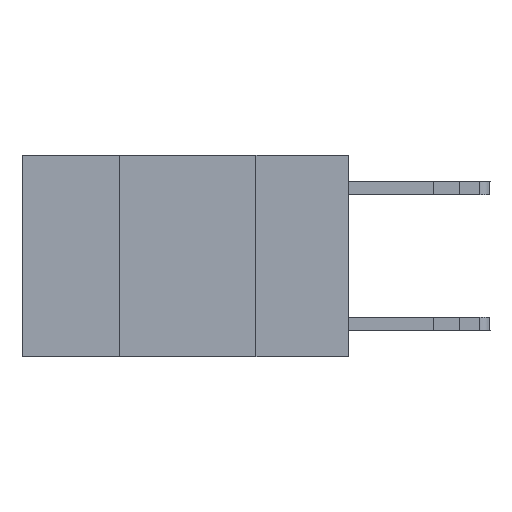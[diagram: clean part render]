
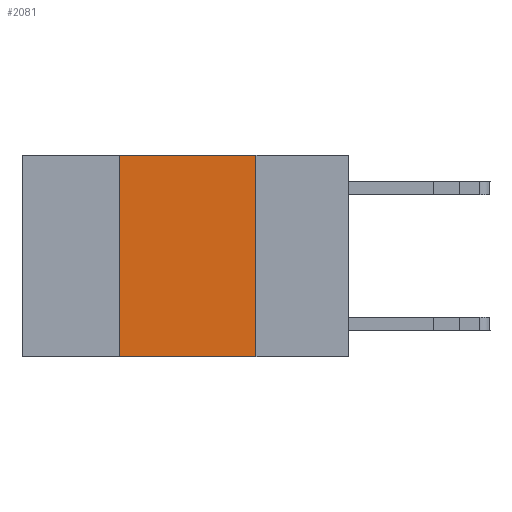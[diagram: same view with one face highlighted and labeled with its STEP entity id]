
A CAD part, left-side view. The second image highlights one B-rep face of the part: STEP entity #2081.
In plain terms, the highlighted planar face has unit normal (-1, 0, 0).
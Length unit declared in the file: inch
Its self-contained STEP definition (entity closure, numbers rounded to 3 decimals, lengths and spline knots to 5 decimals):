
#40 = LINE ( 'NONE', #5530, #3057 ) ;
#93 = CARTESIAN_POINT ( 'NONE',  ( 0., 0.17, -0.37 ) ) ;
#154 = VECTOR ( 'NONE', #2727, 39.37008 ) ;
#348 = EDGE_LOOP ( 'NONE', ( #658, #7552, #931, #5049 ) ) ;
#658 = ORIENTED_EDGE ( 'NONE', *, *, #816, .F. ) ;
#706 = VECTOR ( 'NONE', #5770, 39.37008 ) ;
#811 = DIRECTION ( 'NONE',  ( 1., 0., 0. ) ) ;
#816 = EDGE_CURVE ( 'NONE', #6976, #3836, #6432, .T. ) ;
#931 = ORIENTED_EDGE ( 'NONE', *, *, #13270, .F. ) ;
#2059 = DIRECTION ( 'NONE',  ( 0., 0., -1. ) ) ;
#2081 = ADVANCED_FACE ( 'NONE', ( #9337 ), #7507, .F. ) ;
#2727 = DIRECTION ( 'NONE',  ( 0., -1., 0. ) ) ;
#2883 = CARTESIAN_POINT ( 'NONE',  ( 0., 0.42, 0. ) ) ;
#3057 = VECTOR ( 'NONE', #11741, 39.37008 ) ;
#3382 = LINE ( 'NONE', #13385, #154 ) ;
#3836 = VERTEX_POINT ( 'NONE', #93 ) ;
#4446 = AXIS2_PLACEMENT_3D ( 'NONE', #12583, #811, #10668 ) ;
#5049 = ORIENTED_EDGE ( 'NONE', *, *, #7826, .T. ) ;
#5530 = CARTESIAN_POINT ( 'NONE',  ( 0., 0.6, 0. ) ) ;
#5770 = DIRECTION ( 'NONE',  ( 0., 0., 1. ) ) ;
#6432 = LINE ( 'NONE', #7615, #8735 ) ;
#6503 = EDGE_CURVE ( 'NONE', #11081, #6976, #40, .T. ) ;
#6976 = VERTEX_POINT ( 'NONE', #11138 ) ;
#7257 = CARTESIAN_POINT ( 'NONE',  ( 0., 0.42, 0. ) ) ;
#7507 = PLANE ( 'NONE',  #4446 ) ;
#7552 = ORIENTED_EDGE ( 'NONE', *, *, #6503, .F. ) ;
#7615 = CARTESIAN_POINT ( 'NONE',  ( 0., 0.17, 0. ) ) ;
#7826 = EDGE_CURVE ( 'NONE', #11530, #3836, #3382, .T. ) ;
#8174 = LINE ( 'NONE', #2883, #706 ) ;
#8735 = VECTOR ( 'NONE', #2059, 39.37008 ) ;
#9337 = FACE_OUTER_BOUND ( 'NONE', #348, .T. ) ;
#10668 = DIRECTION ( 'NONE',  ( 0., 0., -1. ) ) ;
#11081 = VERTEX_POINT ( 'NONE', #7257 ) ;
#11138 = CARTESIAN_POINT ( 'NONE',  ( 0., 0.17, 0. ) ) ;
#11530 = VERTEX_POINT ( 'NONE', #13689 ) ;
#11741 = DIRECTION ( 'NONE',  ( 0., -1., 0. ) ) ;
#12583 = CARTESIAN_POINT ( 'NONE',  ( 0., 0.6, 0. ) ) ;
#13270 = EDGE_CURVE ( 'NONE', #11530, #11081, #8174, .T. ) ;
#13385 = CARTESIAN_POINT ( 'NONE',  ( 0., 0.6, -0.37 ) ) ;
#13689 = CARTESIAN_POINT ( 'NONE',  ( 0., 0.42, -0.37 ) ) ;
